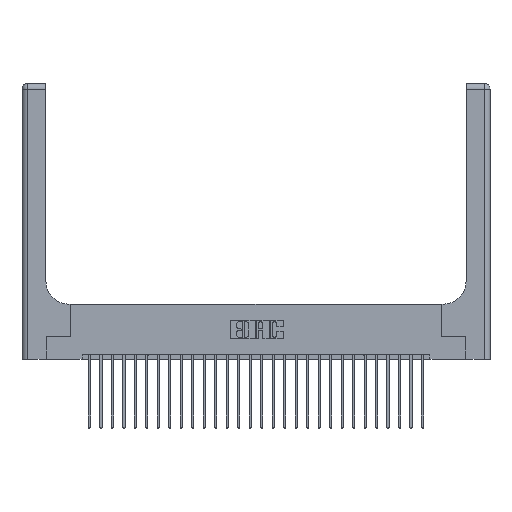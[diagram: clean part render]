
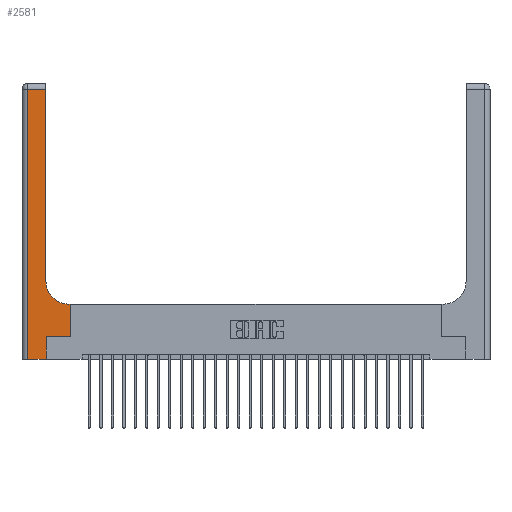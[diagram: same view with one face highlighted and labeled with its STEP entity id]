
A CAD part, top view. The second image highlights one B-rep face of the part: STEP entity #2581.
In plain terms, the highlighted planar face has unit normal (0, 0, 1).
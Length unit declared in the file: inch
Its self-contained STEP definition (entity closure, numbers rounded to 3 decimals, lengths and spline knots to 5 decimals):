
#662 = VECTOR ( 'NONE', #18447, 39.37008 ) ;
#854 = DIRECTION ( 'NONE',  ( 1., 0., 0. ) ) ;
#1141 = EDGE_CURVE ( 'NONE', #5639, #5485, #20609, .T. ) ;
#1475 = CARTESIAN_POINT ( 'NONE',  ( 0.265, 0.25, 0.37 ) ) ;
#1664 = VECTOR ( 'NONE', #21054, 39.37008 ) ;
#1891 = ORIENTED_EDGE ( 'NONE', *, *, #9329, .T. ) ;
#2112 = ORIENTED_EDGE ( 'NONE', *, *, #15346, .T. ) ;
#2581 = ADVANCED_FACE ( 'NONE', ( #12312 ), #15037, .F. ) ;
#3325 = VERTEX_POINT ( 'NONE', #26257 ) ;
#3509 = DIRECTION ( 'NONE',  ( 1., 0., 0. ) ) ;
#3776 = DIRECTION ( 'NONE',  ( 0., 1., 0. ) ) ;
#3837 = EDGE_CURVE ( 'NONE', #22700, #21719, #14171, .T. ) ;
#3991 = VECTOR ( 'NONE', #19113, 39.37008 ) ;
#4190 = CARTESIAN_POINT ( 'NONE',  ( 0.06, 2.94, 0.37 ) ) ;
#4296 = CARTESIAN_POINT ( 'NONE',  ( 0.528, 0.25, 0.37 ) ) ;
#5369 = CARTESIAN_POINT ( 'NONE',  ( 0.51, 0.6, 0.37 ) ) ;
#5485 = VERTEX_POINT ( 'NONE', #13048 ) ;
#5639 = VERTEX_POINT ( 'NONE', #5369 ) ;
#6300 = AXIS2_PLACEMENT_3D ( 'NONE', #11005, #25246, #854 ) ;
#6628 = AXIS2_PLACEMENT_3D ( 'NONE', #16823, #18997, #10813 ) ;
#6691 = VERTEX_POINT ( 'NONE', #23408 ) ;
#6737 = VECTOR ( 'NONE', #20634, 39.37008 ) ;
#8243 = CARTESIAN_POINT ( 'NONE',  ( 0., 2.94, 0.37 ) ) ;
#8282 = LINE ( 'NONE', #9838, #23897 ) ;
#8698 = VECTOR ( 'NONE', #16416, 39.37008 ) ;
#9154 = ORIENTED_EDGE ( 'NONE', *, *, #18065, .T. ) ;
#9329 = EDGE_CURVE ( 'NONE', #6691, #5639, #23975, .T. ) ;
#9838 = CARTESIAN_POINT ( 'NONE',  ( 0.26, 3., 0.37 ) ) ;
#10184 = CARTESIAN_POINT ( 'NONE',  ( 0.265, 0., 0.37 ) ) ;
#10813 = DIRECTION ( 'NONE',  ( -1., 0., 0. ) ) ;
#11005 = CARTESIAN_POINT ( 'NONE',  ( 0.51, 0.85, 0.37 ) ) ;
#11915 = VERTEX_POINT ( 'NONE', #23440 ) ;
#12126 = CARTESIAN_POINT ( 'NONE',  ( 0.528, 0.25, 0.37 ) ) ;
#12273 = DIRECTION ( 'NONE',  ( -1., 0., 0. ) ) ;
#12312 = FACE_OUTER_BOUND ( 'NONE', #17070, .T. ) ;
#13048 = CARTESIAN_POINT ( 'NONE',  ( 0.26, 0.85, 0.37 ) ) ;
#13373 = LINE ( 'NONE', #1475, #17227 ) ;
#14171 = LINE ( 'NONE', #24129, #8698 ) ;
#14289 = ORIENTED_EDGE ( 'NONE', *, *, #25530, .T. ) ;
#14467 = LINE ( 'NONE', #18864, #6737 ) ;
#14871 = LINE ( 'NONE', #25002, #3991 ) ;
#15037 = PLANE ( 'NONE',  #6628 ) ;
#15346 = EDGE_CURVE ( 'NONE', #3325, #22437, #13373, .T. ) ;
#15477 = EDGE_CURVE ( 'NONE', #5485, #11915, #8282, .T. ) ;
#15916 = ORIENTED_EDGE ( 'NONE', *, *, #22219, .T. ) ;
#16416 = DIRECTION ( 'NONE',  ( 1., 0., 0. ) ) ;
#16823 = CARTESIAN_POINT ( 'NONE',  ( 0., 3., 0.37 ) ) ;
#17070 = EDGE_LOOP ( 'NONE', ( #22387, #15916, #9154, #19505, #22364, #2112, #14289, #1891, #17889 ) ) ;
#17103 = LINE ( 'NONE', #8243, #18663 ) ;
#17227 = VECTOR ( 'NONE', #3509, 39.37008 ) ;
#17889 = ORIENTED_EDGE ( 'NONE', *, *, #1141, .T. ) ;
#18065 = EDGE_CURVE ( 'NONE', #24497, #22700, #14871, .T. ) ;
#18447 = DIRECTION ( 'NONE',  ( 0., 1., 0. ) ) ;
#18663 = VECTOR ( 'NONE', #12273, 39.37008 ) ;
#18864 = CARTESIAN_POINT ( 'NONE',  ( 0.265, 0., 0.37 ) ) ;
#18997 = DIRECTION ( 'NONE',  ( 0., 0., -1. ) ) ;
#19113 = DIRECTION ( 'NONE',  ( 0., -1., 0. ) ) ;
#19505 = ORIENTED_EDGE ( 'NONE', *, *, #3837, .T. ) ;
#20609 = CIRCLE ( 'NONE', #6300, 0.25 ) ;
#20634 = DIRECTION ( 'NONE',  ( 0., 1., 0. ) ) ;
#21054 = DIRECTION ( 'NONE',  ( -1., 0., 0. ) ) ;
#21719 = VERTEX_POINT ( 'NONE', #10184 ) ;
#21734 = CARTESIAN_POINT ( 'NONE',  ( 0.06, 0., 0.37 ) ) ;
#22005 = LINE ( 'NONE', #12126, #662 ) ;
#22219 = EDGE_CURVE ( 'NONE', #11915, #24497, #17103, .T. ) ;
#22364 = ORIENTED_EDGE ( 'NONE', *, *, #24643, .T. ) ;
#22387 = ORIENTED_EDGE ( 'NONE', *, *, #15477, .T. ) ;
#22437 = VERTEX_POINT ( 'NONE', #4296 ) ;
#22700 = VERTEX_POINT ( 'NONE', #21734 ) ;
#23408 = CARTESIAN_POINT ( 'NONE',  ( 0.528, 0.6, 0.37 ) ) ;
#23440 = CARTESIAN_POINT ( 'NONE',  ( 0.26, 2.94, 0.37 ) ) ;
#23897 = VECTOR ( 'NONE', #3776, 39.37008 ) ;
#23975 = LINE ( 'NONE', #25440, #1664 ) ;
#24129 = CARTESIAN_POINT ( 'NONE',  ( 0., 0., 0.37 ) ) ;
#24497 = VERTEX_POINT ( 'NONE', #4190 ) ;
#24643 = EDGE_CURVE ( 'NONE', #21719, #3325, #14467, .T. ) ;
#25002 = CARTESIAN_POINT ( 'NONE',  ( 0.06, 3., 0.37 ) ) ;
#25246 = DIRECTION ( 'NONE',  ( 0., 0., -1. ) ) ;
#25440 = CARTESIAN_POINT ( 'NONE',  ( 0.26, 0.6, 0.37 ) ) ;
#25530 = EDGE_CURVE ( 'NONE', #22437, #6691, #22005, .T. ) ;
#26257 = CARTESIAN_POINT ( 'NONE',  ( 0.265, 0.25, 0.37 ) ) ;
